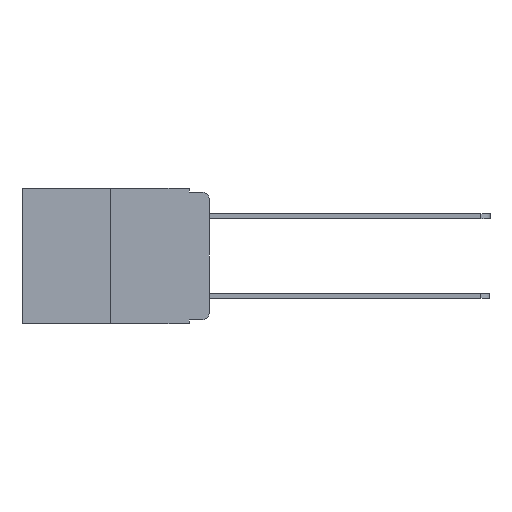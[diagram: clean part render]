
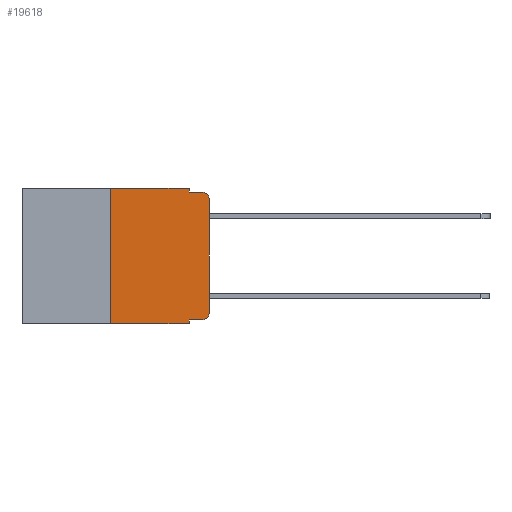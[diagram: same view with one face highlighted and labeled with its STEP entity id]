
A CAD part, left-side view. The second image highlights one B-rep face of the part: STEP entity #19618.
In plain terms, the highlighted planar face has unit normal (-1, 0, 0).
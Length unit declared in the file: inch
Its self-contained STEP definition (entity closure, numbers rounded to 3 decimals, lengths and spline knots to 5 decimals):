
#86 = LINE ( 'NONE', #10401, #15852 ) ;
#206 = CARTESIAN_POINT ( 'NONE',  ( 0., 0.473, 0. ) ) ;
#234 = CARTESIAN_POINT ( 'NONE',  ( 0., 0.051, -0.333 ) ) ;
#283 = VECTOR ( 'NONE', #8790, 39.37008 ) ;
#392 = ORIENTED_EDGE ( 'NONE', *, *, #1530, .T. ) ;
#408 = CARTESIAN_POINT ( 'NONE',  ( 0., 0.02, -0.01 ) ) ;
#416 = VECTOR ( 'NONE', #3428, 39.37008 ) ;
#569 = AXIS2_PLACEMENT_3D ( 'NONE', #1421, #12164, #2961 ) ;
#933 = VERTEX_POINT ( 'NONE', #1644 ) ;
#962 = EDGE_LOOP ( 'NONE', ( #392, #17059, #1843, #14515, #2781, #3265, #11920, #1125, #18261, #3022 ) ) ;
#975 = LINE ( 'NONE', #8100, #4569 ) ;
#1125 = ORIENTED_EDGE ( 'NONE', *, *, #1744, .F. ) ;
#1242 = DIRECTION ( 'NONE',  ( 0., 0., 1. ) ) ;
#1421 = CARTESIAN_POINT ( 'NONE',  ( 0., 0.02, -0.03 ) ) ;
#1530 = EDGE_CURVE ( 'NONE', #933, #19078, #6624, .T. ) ;
#1601 = EDGE_CURVE ( 'NONE', #10764, #933, #5647, .T. ) ;
#1644 = CARTESIAN_POINT ( 'NONE',  ( 0., 0., -0.313 ) ) ;
#1744 = EDGE_CURVE ( 'NONE', #12423, #8054, #86, .T. ) ;
#1788 = VECTOR ( 'NONE', #1242, 39.37008 ) ;
#1843 = ORIENTED_EDGE ( 'NONE', *, *, #9134, .F. ) ;
#2088 = AXIS2_PLACEMENT_3D ( 'NONE', #9498, #15490, #6410 ) ;
#2202 = VERTEX_POINT ( 'NONE', #10430 ) ;
#2502 = VECTOR ( 'NONE', #10960, 39.37008 ) ;
#2616 = DIRECTION ( 'NONE',  ( 1., 0., 0. ) ) ;
#2781 = ORIENTED_EDGE ( 'NONE', *, *, #12677, .F. ) ;
#2838 = CARTESIAN_POINT ( 'NONE',  ( 0., 0.25, 0. ) ) ;
#2961 = DIRECTION ( 'NONE',  ( 0., 0., -1. ) ) ;
#3022 = ORIENTED_EDGE ( 'NONE', *, *, #1601, .T. ) ;
#3265 = ORIENTED_EDGE ( 'NONE', *, *, #8135, .F. ) ;
#3428 = DIRECTION ( 'NONE',  ( 0., -1., 0. ) ) ;
#4569 = VECTOR ( 'NONE', #6540, 39.37008 ) ;
#5178 = VERTEX_POINT ( 'NONE', #18787 ) ;
#5605 = VECTOR ( 'NONE', #14029, 39.37008 ) ;
#5647 = CIRCLE ( 'NONE', #2088, 0.02 ) ;
#6125 = VERTEX_POINT ( 'NONE', #16050 ) ;
#6410 = DIRECTION ( 'NONE',  ( 0., 0., -1. ) ) ;
#6443 = CARTESIAN_POINT ( 'NONE',  ( 0., 0.051, 0. ) ) ;
#6540 = DIRECTION ( 'NONE',  ( 0., -1., 0. ) ) ;
#6608 = LINE ( 'NONE', #6443, #13739 ) ;
#6624 = LINE ( 'NONE', #16849, #2502 ) ;
#7230 = CARTESIAN_POINT ( 'NONE',  ( 0., 0.051, -0.01 ) ) ;
#8054 = VERTEX_POINT ( 'NONE', #16306 ) ;
#8100 = CARTESIAN_POINT ( 'NONE',  ( 0., 0.473, -0.343 ) ) ;
#8135 = EDGE_CURVE ( 'NONE', #6125, #5178, #17475, .T. ) ;
#8347 = EDGE_CURVE ( 'NONE', #2202, #19098, #6608, .T. ) ;
#8790 = DIRECTION ( 'NONE',  ( 0., -1., 0. ) ) ;
#8833 = EDGE_CURVE ( 'NONE', #12423, #10764, #9703, .T. ) ;
#8976 = CARTESIAN_POINT ( 'NONE',  ( 0., 0., -0.03 ) ) ;
#9039 = CARTESIAN_POINT ( 'NONE',  ( 0., 0.051, -0.01 ) ) ;
#9134 = EDGE_CURVE ( 'NONE', #19098, #15342, #13475, .T. ) ;
#9498 = CARTESIAN_POINT ( 'NONE',  ( 0., 0.02, -0.313 ) ) ;
#9703 = LINE ( 'NONE', #234, #5605 ) ;
#9737 = CARTESIAN_POINT ( 'NONE',  ( 0., 0.02, -0.333 ) ) ;
#10109 = CARTESIAN_POINT ( 'NONE',  ( 0., 0.051, -0.333 ) ) ;
#10401 = CARTESIAN_POINT ( 'NONE',  ( 0., 0.051, 0. ) ) ;
#10430 = CARTESIAN_POINT ( 'NONE',  ( 0., 0.051, 0. ) ) ;
#10764 = VERTEX_POINT ( 'NONE', #9737 ) ;
#10960 = DIRECTION ( 'NONE',  ( 0., 0., 1. ) ) ;
#11821 = CARTESIAN_POINT ( 'NONE',  ( 0., 0.473, 0. ) ) ;
#11920 = ORIENTED_EDGE ( 'NONE', *, *, #18069, .T. ) ;
#12164 = DIRECTION ( 'NONE',  ( -1., 0., 0. ) ) ;
#12423 = VERTEX_POINT ( 'NONE', #10109 ) ;
#12448 = FACE_OUTER_BOUND ( 'NONE', #962, .T. ) ;
#12473 = CIRCLE ( 'NONE', #569, 0.02 ) ;
#12677 = EDGE_CURVE ( 'NONE', #5178, #2202, #16614, .T. ) ;
#13352 = DIRECTION ( 'NONE',  ( 0., 0., -1. ) ) ;
#13475 = LINE ( 'NONE', #7230, #283 ) ;
#13739 = VECTOR ( 'NONE', #15521, 39.37008 ) ;
#14029 = DIRECTION ( 'NONE',  ( 0., -1., 0. ) ) ;
#14515 = ORIENTED_EDGE ( 'NONE', *, *, #8347, .F. ) ;
#15342 = VERTEX_POINT ( 'NONE', #408 ) ;
#15490 = DIRECTION ( 'NONE',  ( -1., 0., 0. ) ) ;
#15521 = DIRECTION ( 'NONE',  ( 0., 0., -1. ) ) ;
#15852 = VECTOR ( 'NONE', #16889, 39.37008 ) ;
#16050 = CARTESIAN_POINT ( 'NONE',  ( 0., 0.25, -0.343 ) ) ;
#16306 = CARTESIAN_POINT ( 'NONE',  ( 0., 0.051, -0.343 ) ) ;
#16614 = LINE ( 'NONE', #206, #416 ) ;
#16849 = CARTESIAN_POINT ( 'NONE',  ( 0., 0., 0. ) ) ;
#16889 = DIRECTION ( 'NONE',  ( 0., 0., -1. ) ) ;
#17059 = ORIENTED_EDGE ( 'NONE', *, *, #19109, .T. ) ;
#17475 = LINE ( 'NONE', #2838, #1788 ) ;
#17530 = AXIS2_PLACEMENT_3D ( 'NONE', #11821, #2616, #13352 ) ;
#18069 = EDGE_CURVE ( 'NONE', #6125, #8054, #975, .T. ) ;
#18261 = ORIENTED_EDGE ( 'NONE', *, *, #8833, .T. ) ;
#18787 = CARTESIAN_POINT ( 'NONE',  ( 0., 0.25, 0. ) ) ;
#19078 = VERTEX_POINT ( 'NONE', #8976 ) ;
#19098 = VERTEX_POINT ( 'NONE', #9039 ) ;
#19109 = EDGE_CURVE ( 'NONE', #19078, #15342, #12473, .T. ) ;
#19221 = PLANE ( 'NONE',  #17530 ) ;
#19618 = ADVANCED_FACE ( 'NONE', ( #12448 ), #19221, .F. ) ;
